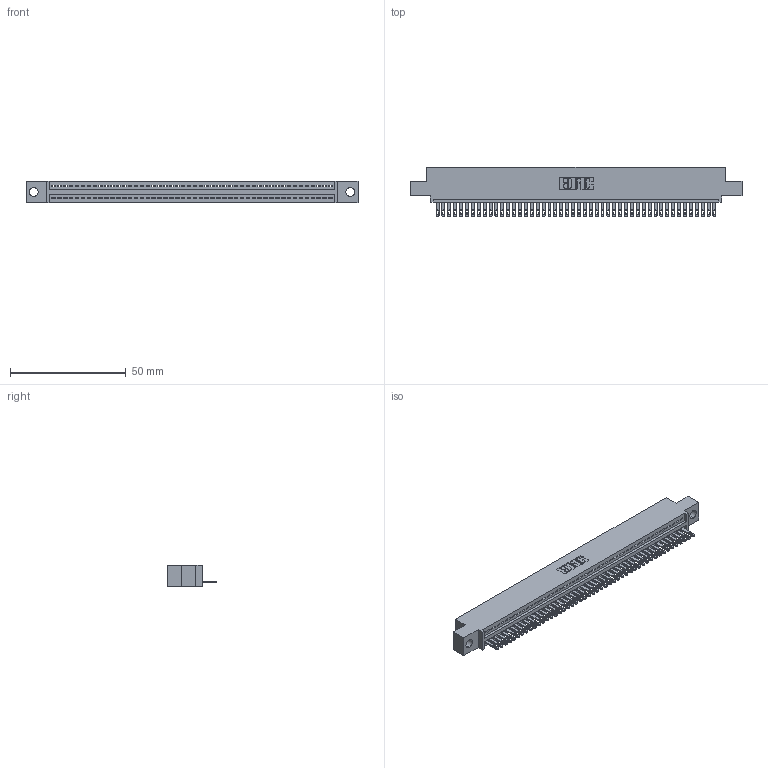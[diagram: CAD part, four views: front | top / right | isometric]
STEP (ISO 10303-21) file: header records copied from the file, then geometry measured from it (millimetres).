
FILE_DESCRIPTION (( 'STEP AP203' ), '1' );
FILE_NAME ('345-048-500-404.STEP', '2021-05-26T15:14:57', ( '' ), ( '' ), 'SwSTEP 2.0', 'SolidWorks 2020', '' );
FILE_SCHEMA (( 'CONFIG_CONTROL_DESIGN' ));
Length unit declared in the file: inch
Products named in the file (3): 345-048-500-404; 345 Part_0.110 Offset - 0.156 Dia-TI; 345-292-001_345-293-100
Assembly tree (49 placements, depth 2):
  345-048-500-404
    345 Part_0.110 Offset - 0.156 Dia-TI
    345-292-001_345-293-100  x48
Bounding box: 143.13 x 21.51 x 9.4 mm (x, y, z)
Volume: 13494.1 mm3; surface area: 18046.1 mm2
Topology: 49 solids, 49 shells, 2736 faces, 8453 edges, 5634 vertices
Faces by surface type: plane 1730, cylinder 1006
Entity records: 35799 total; most frequent: CARTESIAN_POINT 6210, ORIENTED_EDGE 6190, DIRECTION 5415, EDGE_CURVE 3095, VECTOR 2767, LINE 2767, VERTEX_POINT 2062, AXIS2_PLACEMENT_3D 1324
